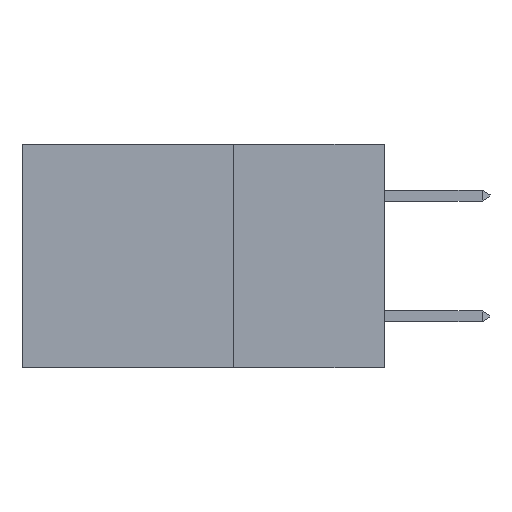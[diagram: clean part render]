
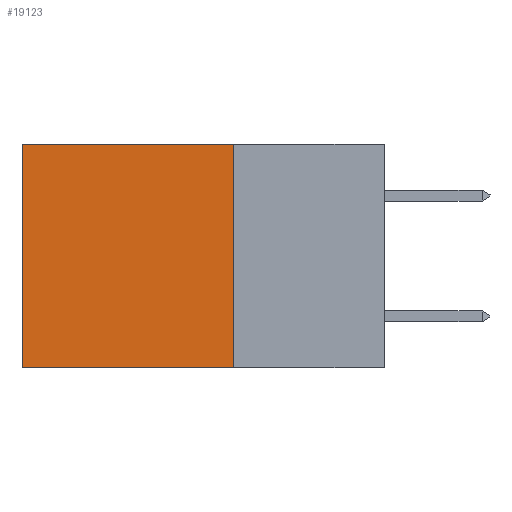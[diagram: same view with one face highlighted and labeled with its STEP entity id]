
A CAD part, left-side view. The second image highlights one B-rep face of the part: STEP entity #19123.
In plain terms, the highlighted planar face has unit normal (-1, 0, 0).
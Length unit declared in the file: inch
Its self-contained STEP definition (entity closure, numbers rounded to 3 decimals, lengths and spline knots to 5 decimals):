
#133 = EDGE_CURVE ( 'NONE', #33946, #2070, #12613, .T. ) ;
#359 = CARTESIAN_POINT ( 'NONE',  ( 0.2875, 0.6, 0. ) ) ;
#1345 = ORIENTED_EDGE ( 'NONE', *, *, #7683, .T. ) ;
#2070 = VERTEX_POINT ( 'NONE', #12020 ) ;
#2567 = CARTESIAN_POINT ( 'NONE',  ( 0.2875, 0.25, 0. ) ) ;
#3594 = FACE_OUTER_BOUND ( 'NONE', #30712, .T. ) ;
#6675 = VECTOR ( 'NONE', #43748, 39.37008 ) ;
#7683 = EDGE_CURVE ( 'NONE', #33946, #12569, #39197, .T. ) ;
#8078 = CARTESIAN_POINT ( 'NONE',  ( 0.2875, 0.25, 0. ) ) ;
#8710 = AXIS2_PLACEMENT_3D ( 'NONE', #17843, #24660, #31502 ) ;
#9270 = DIRECTION ( 'NONE',  ( 0., 1., 0. ) ) ;
#11534 = DIRECTION ( 'NONE',  ( 0., 0., -1. ) ) ;
#12020 = CARTESIAN_POINT ( 'NONE',  ( 0.2875, 0.25, -0.37 ) ) ;
#12352 = LINE ( 'NONE', #359, #41664 ) ;
#12569 = VERTEX_POINT ( 'NONE', #19889 ) ;
#12613 = LINE ( 'NONE', #8078, #15795 ) ;
#15795 = VECTOR ( 'NONE', #11534, 39.37008 ) ;
#16927 = CARTESIAN_POINT ( 'NONE',  ( 0.2875, 0.25, 0. ) ) ;
#17359 = CARTESIAN_POINT ( 'NONE',  ( 0.2875, 0.6, -0.37 ) ) ;
#17843 = CARTESIAN_POINT ( 'NONE',  ( 0.2875, 0.25, 0. ) ) ;
#19123 = ADVANCED_FACE ( 'NONE', ( #3594 ), #31351, .F. ) ;
#19889 = CARTESIAN_POINT ( 'NONE',  ( 0.2875, 0.6, 0. ) ) ;
#20132 = DIRECTION ( 'NONE',  ( 0., 0., -1. ) ) ;
#24660 = DIRECTION ( 'NONE',  ( 1., 0., 0. ) ) ;
#25495 = EDGE_CURVE ( 'NONE', #2070, #36788, #34673, .T. ) ;
#27582 = ORIENTED_EDGE ( 'NONE', *, *, #29072, .T. ) ;
#28621 = VECTOR ( 'NONE', #9270, 39.37008 ) ;
#29072 = EDGE_CURVE ( 'NONE', #12569, #36788, #12352, .T. ) ;
#29582 = ORIENTED_EDGE ( 'NONE', *, *, #25495, .F. ) ;
#30712 = EDGE_LOOP ( 'NONE', ( #27582, #29582, #41216, #1345 ) ) ;
#31351 = PLANE ( 'NONE',  #8710 ) ;
#31502 = DIRECTION ( 'NONE',  ( 0., 0., -1. ) ) ;
#33946 = VERTEX_POINT ( 'NONE', #2567 ) ;
#34673 = LINE ( 'NONE', #43259, #28621 ) ;
#36788 = VERTEX_POINT ( 'NONE', #17359 ) ;
#39197 = LINE ( 'NONE', #16927, #6675 ) ;
#41216 = ORIENTED_EDGE ( 'NONE', *, *, #133, .F. ) ;
#41664 = VECTOR ( 'NONE', #20132, 39.37008 ) ;
#43259 = CARTESIAN_POINT ( 'NONE',  ( 0.2875, 0.25, -0.37 ) ) ;
#43748 = DIRECTION ( 'NONE',  ( 0., 1., 0. ) ) ;
